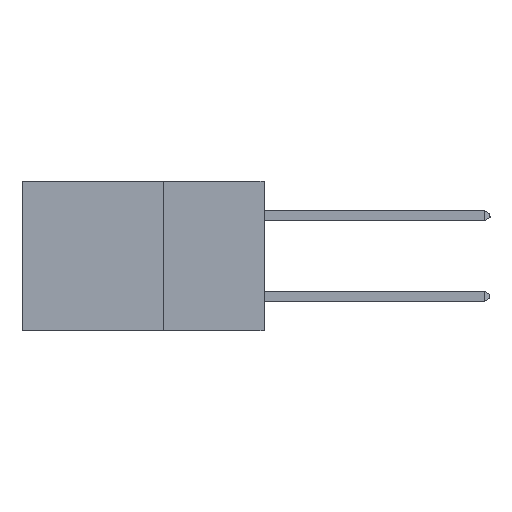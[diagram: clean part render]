
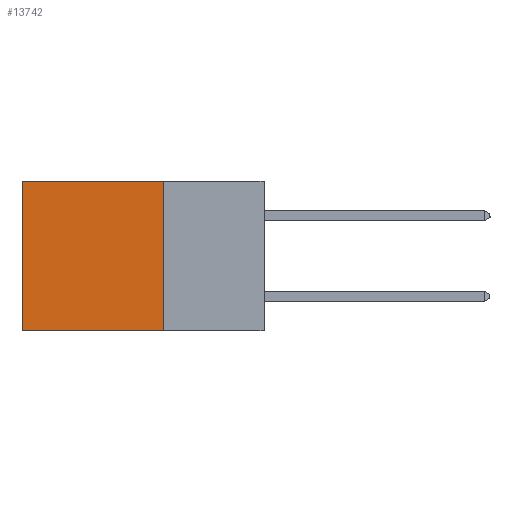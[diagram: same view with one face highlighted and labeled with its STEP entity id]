
A CAD part, left-side view. The second image highlights one B-rep face of the part: STEP entity #13742.
In plain terms, the highlighted planar face has unit normal (-1, 0, 0).
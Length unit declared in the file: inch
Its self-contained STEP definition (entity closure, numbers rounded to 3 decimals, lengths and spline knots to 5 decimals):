
#554 = VERTEX_POINT ( 'NONE', #9282 ) ;
#1062 = VERTEX_POINT ( 'NONE', #10817 ) ;
#2181 = CARTESIAN_POINT ( 'NONE',  ( 0.298, 0.25, -0.37 ) ) ;
#2243 = CARTESIAN_POINT ( 'NONE',  ( 0.298, 0.25, 0. ) ) ;
#3139 = FACE_OUTER_BOUND ( 'NONE', #9081, .T. ) ;
#3795 = VERTEX_POINT ( 'NONE', #3932 ) ;
#3898 = CARTESIAN_POINT ( 'NONE',  ( 0.298, 0.25, 0. ) ) ;
#3932 = CARTESIAN_POINT ( 'NONE',  ( 0.298, 0.6, 0. ) ) ;
#4279 = CARTESIAN_POINT ( 'NONE',  ( 0.298, 0.25, -0.37 ) ) ;
#4933 = CARTESIAN_POINT ( 'NONE',  ( 0.298, 0.6, 0. ) ) ;
#5096 = EDGE_CURVE ( 'NONE', #12912, #1062, #20446, .T. ) ;
#5647 = DIRECTION ( 'NONE',  ( 0., 0., -1. ) ) ;
#6807 = ORIENTED_EDGE ( 'NONE', *, *, #9005, .T. ) ;
#6962 = LINE ( 'NONE', #2243, #11872 ) ;
#7411 = ORIENTED_EDGE ( 'NONE', *, *, #12254, .T. ) ;
#7532 = VECTOR ( 'NONE', #8211, 39.37008 ) ;
#8211 = DIRECTION ( 'NONE',  ( 0., 0., -1. ) ) ;
#8627 = ORIENTED_EDGE ( 'NONE', *, *, #5096, .F. ) ;
#9005 = EDGE_CURVE ( 'NONE', #3795, #1062, #16860, .T. ) ;
#9081 = EDGE_LOOP ( 'NONE', ( #6807, #8627, #15519, #7411 ) ) ;
#9282 = CARTESIAN_POINT ( 'NONE',  ( 0.298, 0.25, 0. ) ) ;
#10817 = CARTESIAN_POINT ( 'NONE',  ( 0.298, 0.6, -0.37 ) ) ;
#11872 = VECTOR ( 'NONE', #13949, 39.37008 ) ;
#12254 = EDGE_CURVE ( 'NONE', #554, #3795, #6962, .T. ) ;
#12461 = LINE ( 'NONE', #14134, #20148 ) ;
#12912 = VERTEX_POINT ( 'NONE', #4279 ) ;
#13742 = ADVANCED_FACE ( 'NONE', ( #3139 ), #13895, .F. ) ;
#13883 = DIRECTION ( 'NONE',  ( 0., 1., 0. ) ) ;
#13895 = PLANE ( 'NONE',  #16007 ) ;
#13949 = DIRECTION ( 'NONE',  ( 0., 1., 0. ) ) ;
#14134 = CARTESIAN_POINT ( 'NONE',  ( 0.298, 0.25, 0. ) ) ;
#15519 = ORIENTED_EDGE ( 'NONE', *, *, #18737, .F. ) ;
#15594 = DIRECTION ( 'NONE',  ( 1., 0., 0. ) ) ;
#15821 = DIRECTION ( 'NONE',  ( 0., 0., -1. ) ) ;
#16007 = AXIS2_PLACEMENT_3D ( 'NONE', #3898, #15594, #5647 ) ;
#16641 = VECTOR ( 'NONE', #13883, 39.37008 ) ;
#16860 = LINE ( 'NONE', #4933, #7532 ) ;
#18737 = EDGE_CURVE ( 'NONE', #554, #12912, #12461, .T. ) ;
#20148 = VECTOR ( 'NONE', #15821, 39.37008 ) ;
#20446 = LINE ( 'NONE', #2181, #16641 ) ;
